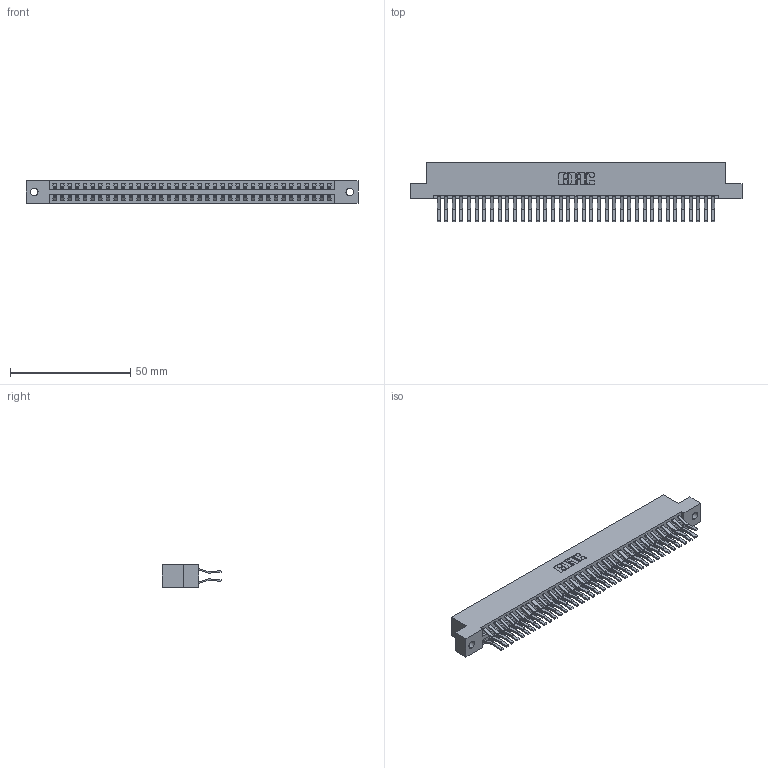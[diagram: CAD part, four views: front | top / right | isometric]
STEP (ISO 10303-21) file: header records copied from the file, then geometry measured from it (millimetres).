
FILE_DESCRIPTION (( 'STEP AP203' ), '1' );
FILE_NAME ('346-074-560-202.STEP', '2018-08-29T03:13:56', ( '' ), ( '' ), 'SwSTEP 2.0', 'SolidWorks 2016', '' );
FILE_SCHEMA (( 'CONFIG_CONTROL_DESIGN' ));
Length unit declared in the file: inch
Products named in the file (3): 345-292-001_560 Tail; 346-074-560-202; 346 Part_Flush Mounting Lugs - 0.128 Dia
Assembly tree (75 placements, depth 2):
  346-074-560-202
    346 Part_Flush Mounting Lugs - 0.128 Dia
    345-292-001_560 Tail  x74
Bounding box: 138.05 x 24.78 x 9.4 mm (x, y, z)
Volume: 13871 mm3; surface area: 20012.9 mm2
Topology: 75 solids, 75 shells, 4118 faces, 12243 edges, 8062 vertices
Faces by surface type: plane 2666, cylinder 1452
Entity records: 24911 total; most frequent: CARTESIAN_POINT 4112, ORIENTED_EDGE 4046, DIRECTION 3679, EDGE_CURVE 2023, VECTOR 1739, LINE 1739, VERTEX_POINT 1346, AXIS2_PLACEMENT_3D 970
